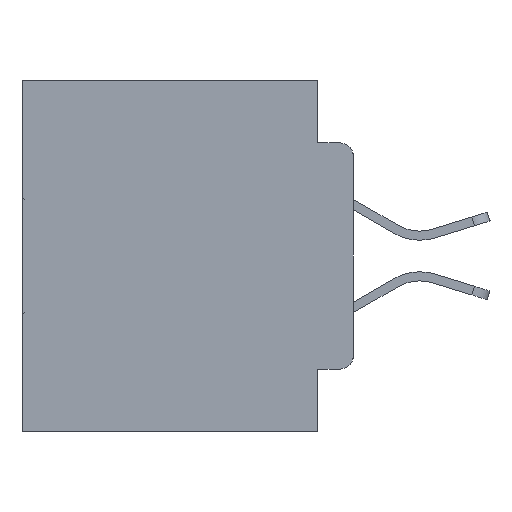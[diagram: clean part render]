
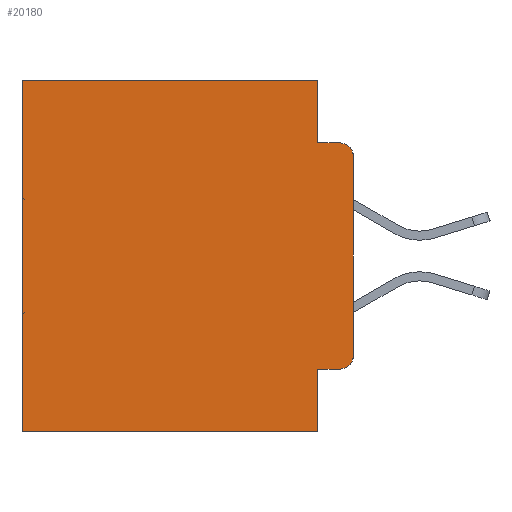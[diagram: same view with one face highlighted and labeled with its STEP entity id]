
A CAD part, left-side view. The second image highlights one B-rep face of the part: STEP entity #20180.
In plain terms, the highlighted planar face has unit normal (-1, 0, 0).
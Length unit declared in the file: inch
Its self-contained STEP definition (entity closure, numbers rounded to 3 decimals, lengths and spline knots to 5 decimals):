
#49 = EDGE_CURVE ( 'NONE', #1913, #18322, #13714, .T. ) ;
#741 = CARTESIAN_POINT ( 'NONE',  ( 0.298, 0.051, 0. ) ) ;
#1423 = EDGE_CURVE ( 'NONE', #28014, #7296, #22444, .T. ) ;
#1628 = ORIENTED_EDGE ( 'NONE', *, *, #49, .T. ) ;
#1913 = VERTEX_POINT ( 'NONE', #11984 ) ;
#2260 = CARTESIAN_POINT ( 'NONE',  ( 0.298, 0.473, 0. ) ) ;
#3102 = VERTEX_POINT ( 'NONE', #6210 ) ;
#3403 = DIRECTION ( 'NONE',  ( 0., 0., -1. ) ) ;
#3875 = CARTESIAN_POINT ( 'NONE',  ( 0.298, 0.02, -0.0885 ) ) ;
#4129 = LINE ( 'NONE', #11569, #7253 ) ;
#4262 = ORIENTED_EDGE ( 'NONE', *, *, #1423, .T. ) ;
#4513 = ORIENTED_EDGE ( 'NONE', *, *, #21430, .F. ) ;
#5449 = ORIENTED_EDGE ( 'NONE', *, *, #6385, .F. ) ;
#5459 = VERTEX_POINT ( 'NONE', #15964 ) ;
#5478 = ORIENTED_EDGE ( 'NONE', *, *, #16323, .T. ) ;
#5916 = LINE ( 'NONE', #17827, #22196 ) ;
#6210 = CARTESIAN_POINT ( 'NONE',  ( 0.298, 0.051, 0. ) ) ;
#6235 = DIRECTION ( 'NONE',  ( 0., 0., -1. ) ) ;
#6385 = EDGE_CURVE ( 'NONE', #30953, #7387, #20679, .T. ) ;
#6814 = PLANE ( 'NONE',  #19464 ) ;
#6915 = EDGE_CURVE ( 'NONE', #24687, #27278, #30144, .T. ) ;
#7253 = VECTOR ( 'NONE', #31366, 39.37008 ) ;
#7296 = VERTEX_POINT ( 'NONE', #3875 ) ;
#7387 = VERTEX_POINT ( 'NONE', #19870 ) ;
#8080 = LINE ( 'NONE', #18134, #9017 ) ;
#8143 = CARTESIAN_POINT ( 'NONE',  ( 0.298, 0.051, 0. ) ) ;
#8499 = VECTOR ( 'NONE', #18520, 39.37008 ) ;
#8729 = CARTESIAN_POINT ( 'NONE',  ( 0.298, 0.473, 0. ) ) ;
#8801 = FACE_OUTER_BOUND ( 'NONE', #27735, .T. ) ;
#8978 = CARTESIAN_POINT ( 'NONE',  ( 0.298, 0.473, -0.5 ) ) ;
#9017 = VECTOR ( 'NONE', #18779, 39.37008 ) ;
#9315 = CARTESIAN_POINT ( 'NONE',  ( 0.298, 0.051, -0.4115 ) ) ;
#11122 = VECTOR ( 'NONE', #28264, 39.37008 ) ;
#11569 = CARTESIAN_POINT ( 'NONE',  ( 0.298, 0.051, -0.4115 ) ) ;
#11795 = VECTOR ( 'NONE', #18407, 39.37008 ) ;
#11984 = CARTESIAN_POINT ( 'NONE',  ( 0.298, 0.02, -0.4115 ) ) ;
#12247 = ORIENTED_EDGE ( 'NONE', *, *, #24499, .F. ) ;
#12453 = AXIS2_PLACEMENT_3D ( 'NONE', #22388, #14830, #24701 ) ;
#13428 = CARTESIAN_POINT ( 'NONE',  ( 0.298, 0., 0. ) ) ;
#13627 = LINE ( 'NONE', #741, #11795 ) ;
#13714 = CIRCLE ( 'NONE', #31091, 0.02 ) ;
#14830 = DIRECTION ( 'NONE',  ( -1., 0., 0. ) ) ;
#15575 = LINE ( 'NONE', #13428, #11122 ) ;
#15964 = CARTESIAN_POINT ( 'NONE',  ( 0.298, 0.051, -0.0885 ) ) ;
#15992 = DIRECTION ( 'NONE',  ( 0., -1., 0. ) ) ;
#16323 = EDGE_CURVE ( 'NONE', #30953, #1913, #4129, .T. ) ;
#17524 = VECTOR ( 'NONE', #18086, 39.37008 ) ;
#17827 = CARTESIAN_POINT ( 'NONE',  ( 0.298, 0.051, -0.0885 ) ) ;
#18086 = DIRECTION ( 'NONE',  ( 0., 0., -1. ) ) ;
#18134 = CARTESIAN_POINT ( 'NONE',  ( 0.298, 0., -0.5 ) ) ;
#18239 = EDGE_CURVE ( 'NONE', #3102, #5459, #13627, .T. ) ;
#18322 = VERTEX_POINT ( 'NONE', #26147 ) ;
#18407 = DIRECTION ( 'NONE',  ( 0., 0., -1. ) ) ;
#18520 = DIRECTION ( 'NONE',  ( 0., 0., -1. ) ) ;
#18611 = CARTESIAN_POINT ( 'NONE',  ( 0.298, 0.02, -0.3915 ) ) ;
#18779 = DIRECTION ( 'NONE',  ( 0., 1., 0. ) ) ;
#18917 = LINE ( 'NONE', #26497, #21793 ) ;
#19464 = AXIS2_PLACEMENT_3D ( 'NONE', #26606, #26278, #23957 ) ;
#19870 = CARTESIAN_POINT ( 'NONE',  ( 0.298, 0.051, -0.5 ) ) ;
#20180 = ADVANCED_FACE ( 'NONE', ( #8801 ), #6814, .F. ) ;
#20679 = LINE ( 'NONE', #8143, #8499 ) ;
#21430 = EDGE_CURVE ( 'NONE', #7387, #27278, #8080, .T. ) ;
#21639 = ORIENTED_EDGE ( 'NONE', *, *, #25678, .T. ) ;
#21793 = VECTOR ( 'NONE', #3403, 39.37008 ) ;
#22196 = VECTOR ( 'NONE', #15992, 39.37008 ) ;
#22388 = CARTESIAN_POINT ( 'NONE',  ( 0.298, 0.02, -0.1085 ) ) ;
#22444 = CIRCLE ( 'NONE', #12453, 0.02 ) ;
#23957 = DIRECTION ( 'NONE',  ( 0., 0., -1. ) ) ;
#24499 = EDGE_CURVE ( 'NONE', #5459, #7296, #5916, .T. ) ;
#24687 = VERTEX_POINT ( 'NONE', #8729 ) ;
#24701 = DIRECTION ( 'NONE',  ( 0., 0., -1. ) ) ;
#25678 = EDGE_CURVE ( 'NONE', #3102, #24687, #15575, .T. ) ;
#26147 = CARTESIAN_POINT ( 'NONE',  ( 0.298, 0., -0.3915 ) ) ;
#26278 = DIRECTION ( 'NONE',  ( 1., 0., 0. ) ) ;
#26497 = CARTESIAN_POINT ( 'NONE',  ( 0.298, 0., 0. ) ) ;
#26525 = DIRECTION ( 'NONE',  ( -1., 0., 0. ) ) ;
#26606 = CARTESIAN_POINT ( 'NONE',  ( 0.298, 0., 0. ) ) ;
#27278 = VERTEX_POINT ( 'NONE', #8978 ) ;
#27735 = EDGE_LOOP ( 'NONE', ( #29531, #4262, #12247, #30219, #21639, #27746, #4513, #5449, #5478, #1628 ) ) ;
#27746 = ORIENTED_EDGE ( 'NONE', *, *, #6915, .T. ) ;
#27874 = CARTESIAN_POINT ( 'NONE',  ( 0.298, 0., -0.1085 ) ) ;
#28014 = VERTEX_POINT ( 'NONE', #27874 ) ;
#28264 = DIRECTION ( 'NONE',  ( 0., 1., 0. ) ) ;
#28604 = EDGE_CURVE ( 'NONE', #28014, #18322, #18917, .T. ) ;
#29531 = ORIENTED_EDGE ( 'NONE', *, *, #28604, .F. ) ;
#30144 = LINE ( 'NONE', #2260, #17524 ) ;
#30219 = ORIENTED_EDGE ( 'NONE', *, *, #18239, .F. ) ;
#30953 = VERTEX_POINT ( 'NONE', #9315 ) ;
#31091 = AXIS2_PLACEMENT_3D ( 'NONE', #18611, #26525, #6235 ) ;
#31366 = DIRECTION ( 'NONE',  ( 0., -1., 0. ) ) ;
